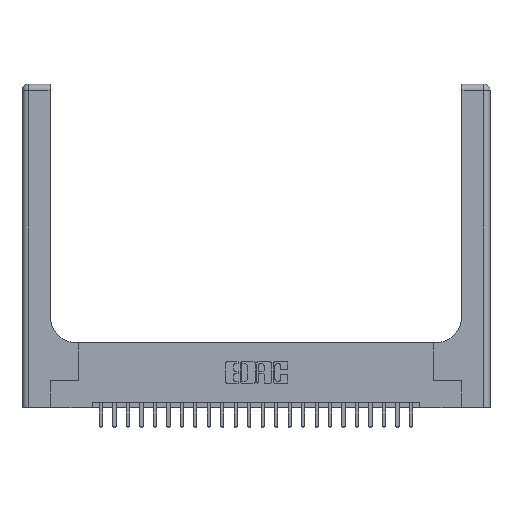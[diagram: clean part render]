
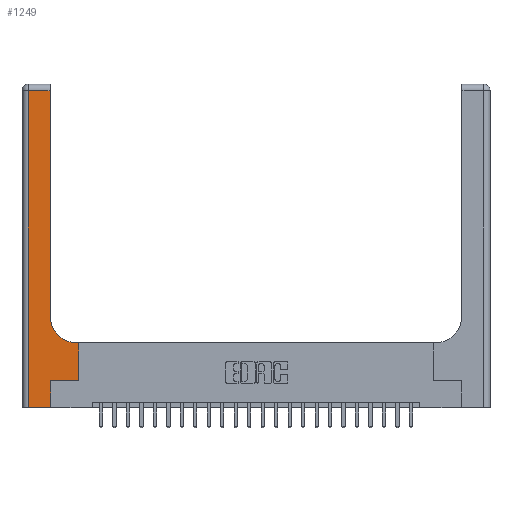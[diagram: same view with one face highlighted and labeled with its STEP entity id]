
A CAD part, top view. The second image highlights one B-rep face of the part: STEP entity #1249.
In plain terms, the highlighted planar face has unit normal (0, 0, 1).
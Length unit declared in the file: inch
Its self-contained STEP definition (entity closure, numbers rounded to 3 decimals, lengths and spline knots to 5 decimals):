
#10 = CARTESIAN_POINT ( 'NONE',  ( 0.265, 0., 0.37 ) ) ;
#33 = CIRCLE ( 'NONE', #22445, 0.25 ) ;
#776 = LINE ( 'NONE', #2260, #12412 ) ;
#863 = VECTOR ( 'NONE', #9252, 39.37008 ) ;
#1249 = ADVANCED_FACE ( 'NONE', ( #15321 ), #15457, .F. ) ;
#2078 = DIRECTION ( 'NONE',  ( 1., 0., 0. ) ) ;
#2260 = CARTESIAN_POINT ( 'NONE',  ( 0.26, 3., 0.37 ) ) ;
#2312 = DIRECTION ( 'NONE',  ( 0., 0., -1. ) ) ;
#2379 = LINE ( 'NONE', #18525, #22123 ) ;
#2434 = CARTESIAN_POINT ( 'NONE',  ( 0.26, 0.6, 0.37 ) ) ;
#3032 = ORIENTED_EDGE ( 'NONE', *, *, #10286, .T. ) ;
#3455 = LINE ( 'NONE', #10, #863 ) ;
#3746 = CARTESIAN_POINT ( 'NONE',  ( 0., 0., 0.37 ) ) ;
#4636 = DIRECTION ( 'NONE',  ( 0., 0., -1. ) ) ;
#5828 = EDGE_CURVE ( 'NONE', #15589, #12320, #16886, .T. ) ;
#5837 = DIRECTION ( 'NONE',  ( 0., 1., 0. ) ) ;
#5994 = VERTEX_POINT ( 'NONE', #17107 ) ;
#6438 = CARTESIAN_POINT ( 'NONE',  ( 0., 3., 0.37 ) ) ;
#6604 = VERTEX_POINT ( 'NONE', #19864 ) ;
#7196 = LINE ( 'NONE', #3746, #18149 ) ;
#7994 = VERTEX_POINT ( 'NONE', #11803 ) ;
#8077 = EDGE_CURVE ( 'NONE', #5994, #19238, #16282, .T. ) ;
#8200 = VECTOR ( 'NONE', #22149, 39.37008 ) ;
#8593 = ORIENTED_EDGE ( 'NONE', *, *, #16995, .T. ) ;
#9252 = DIRECTION ( 'NONE',  ( 0., 1., 0. ) ) ;
#9813 = CARTESIAN_POINT ( 'NONE',  ( 0.26, 2.94, 0.37 ) ) ;
#9942 = ORIENTED_EDGE ( 'NONE', *, *, #8077, .T. ) ;
#10286 = EDGE_CURVE ( 'NONE', #12320, #21730, #2379, .T. ) ;
#10414 = ORIENTED_EDGE ( 'NONE', *, *, #18665, .T. ) ;
#10449 = CARTESIAN_POINT ( 'NONE',  ( 0.528, 0.25, 0.37 ) ) ;
#10943 = CARTESIAN_POINT ( 'NONE',  ( 0.265, 0.25, 0.37 ) ) ;
#11669 = DIRECTION ( 'NONE',  ( -1., 0., 0. ) ) ;
#11803 = CARTESIAN_POINT ( 'NONE',  ( 0.265, 0., 0.37 ) ) ;
#12320 = VERTEX_POINT ( 'NONE', #16670 ) ;
#12412 = VECTOR ( 'NONE', #5837, 39.37008 ) ;
#12595 = DIRECTION ( 'NONE',  ( 1., 0., 0. ) ) ;
#12868 = CARTESIAN_POINT ( 'NONE',  ( 0.26, 0.85, 0.37 ) ) ;
#13158 = CARTESIAN_POINT ( 'NONE',  ( 0.51, 0.85, 0.37 ) ) ;
#13260 = VERTEX_POINT ( 'NONE', #12868 ) ;
#13820 = VECTOR ( 'NONE', #17625, 39.37008 ) ;
#13932 = DIRECTION ( 'NONE',  ( 0., 1., 0. ) ) ;
#14016 = ORIENTED_EDGE ( 'NONE', *, *, #21954, .T. ) ;
#14164 = CARTESIAN_POINT ( 'NONE',  ( 0.06, 0., 0.37 ) ) ;
#14282 = ORIENTED_EDGE ( 'NONE', *, *, #22636, .T. ) ;
#14614 = VECTOR ( 'NONE', #13932, 39.37008 ) ;
#15321 = FACE_OUTER_BOUND ( 'NONE', #15350, .T. ) ;
#15350 = EDGE_LOOP ( 'NONE', ( #16013, #19770, #3032, #18707, #10414, #8593, #9942, #14282, #14016 ) ) ;
#15457 = PLANE ( 'NONE',  #21332 ) ;
#15589 = VERTEX_POINT ( 'NONE', #9813 ) ;
#15666 = CARTESIAN_POINT ( 'NONE',  ( 0.265, 0.25, 0.37 ) ) ;
#16013 = ORIENTED_EDGE ( 'NONE', *, *, #20538, .T. ) ;
#16282 = LINE ( 'NONE', #10449, #14614 ) ;
#16670 = CARTESIAN_POINT ( 'NONE',  ( 0.06, 2.94, 0.37 ) ) ;
#16886 = LINE ( 'NONE', #22799, #13820 ) ;
#16995 = EDGE_CURVE ( 'NONE', #19416, #5994, #21573, .T. ) ;
#17107 = CARTESIAN_POINT ( 'NONE',  ( 0.528, 0.25, 0.37 ) ) ;
#17625 = DIRECTION ( 'NONE',  ( -1., 0., 0. ) ) ;
#17971 = EDGE_CURVE ( 'NONE', #21730, #7994, #7196, .T. ) ;
#18149 = VECTOR ( 'NONE', #12595, 39.37008 ) ;
#18525 = CARTESIAN_POINT ( 'NONE',  ( 0.06, 3., 0.37 ) ) ;
#18665 = EDGE_CURVE ( 'NONE', #7994, #19416, #3455, .T. ) ;
#18707 = ORIENTED_EDGE ( 'NONE', *, *, #17971, .T. ) ;
#19238 = VERTEX_POINT ( 'NONE', #22236 ) ;
#19416 = VERTEX_POINT ( 'NONE', #15666 ) ;
#19731 = LINE ( 'NONE', #2434, #8200 ) ;
#19770 = ORIENTED_EDGE ( 'NONE', *, *, #5828, .T. ) ;
#19864 = CARTESIAN_POINT ( 'NONE',  ( 0.51, 0.6, 0.37 ) ) ;
#19890 = VECTOR ( 'NONE', #21777, 39.37008 ) ;
#20335 = DIRECTION ( 'NONE',  ( 0., -1., 0. ) ) ;
#20538 = EDGE_CURVE ( 'NONE', #13260, #15589, #776, .T. ) ;
#21332 = AXIS2_PLACEMENT_3D ( 'NONE', #6438, #4636, #11669 ) ;
#21573 = LINE ( 'NONE', #10943, #19890 ) ;
#21730 = VERTEX_POINT ( 'NONE', #14164 ) ;
#21777 = DIRECTION ( 'NONE',  ( 1., 0., 0. ) ) ;
#21954 = EDGE_CURVE ( 'NONE', #6604, #13260, #33, .T. ) ;
#22123 = VECTOR ( 'NONE', #20335, 39.37008 ) ;
#22149 = DIRECTION ( 'NONE',  ( -1., 0., 0. ) ) ;
#22236 = CARTESIAN_POINT ( 'NONE',  ( 0.528, 0.6, 0.37 ) ) ;
#22445 = AXIS2_PLACEMENT_3D ( 'NONE', #13158, #2312, #2078 ) ;
#22636 = EDGE_CURVE ( 'NONE', #19238, #6604, #19731, .T. ) ;
#22799 = CARTESIAN_POINT ( 'NONE',  ( 0., 2.94, 0.37 ) ) ;
